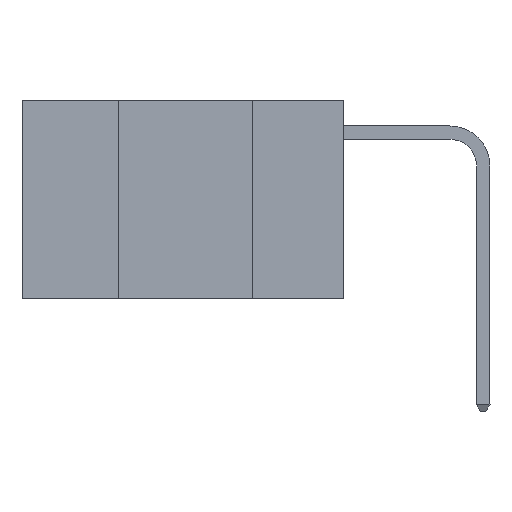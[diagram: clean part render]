
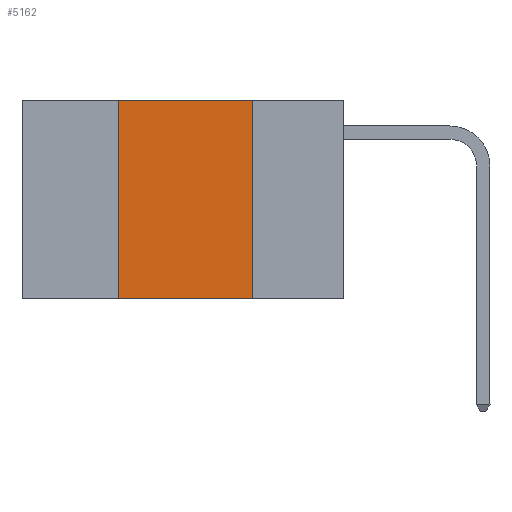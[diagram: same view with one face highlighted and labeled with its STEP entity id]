
A CAD part, left-side view. The second image highlights one B-rep face of the part: STEP entity #5162.
In plain terms, the highlighted planar face has unit normal (-1, 0, 0).
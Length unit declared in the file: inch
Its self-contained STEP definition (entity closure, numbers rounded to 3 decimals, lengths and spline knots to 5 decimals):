
#188 = EDGE_LOOP ( 'NONE', ( #9481, #11231, #2184, #12430 ) ) ;
#251 = CARTESIAN_POINT ( 'NONE',  ( 0., 0.6, -0.37 ) ) ;
#469 = DIRECTION ( 'NONE',  ( 0., 0., 1. ) ) ;
#737 = LINE ( 'NONE', #3701, #4433 ) ;
#960 = VERTEX_POINT ( 'NONE', #8768 ) ;
#1299 = CARTESIAN_POINT ( 'NONE',  ( 0., 0.42, 0. ) ) ;
#1723 = DIRECTION ( 'NONE',  ( 0., 0., -1. ) ) ;
#1767 = VECTOR ( 'NONE', #469, 39.37008 ) ;
#2184 = ORIENTED_EDGE ( 'NONE', *, *, #3793, .F. ) ;
#2724 = DIRECTION ( 'NONE',  ( 0., -1., 0. ) ) ;
#3566 = LINE ( 'NONE', #251, #10297 ) ;
#3701 = CARTESIAN_POINT ( 'NONE',  ( 0., 0.6, 0. ) ) ;
#3793 = EDGE_CURVE ( 'NONE', #13239, #7652, #7542, .T. ) ;
#3947 = CARTESIAN_POINT ( 'NONE',  ( 0., 0.42, -0.37 ) ) ;
#4055 = EDGE_CURVE ( 'NONE', #7652, #960, #737, .T. ) ;
#4138 = CARTESIAN_POINT ( 'NONE',  ( 0., 0.6, 0. ) ) ;
#4433 = VECTOR ( 'NONE', #2724, 39.37008 ) ;
#4456 = DIRECTION ( 'NONE',  ( 0., -1., 0. ) ) ;
#4818 = LINE ( 'NONE', #11314, #11617 ) ;
#5162 = ADVANCED_FACE ( 'NONE', ( #12511 ), #7145, .F. ) ;
#6239 = AXIS2_PLACEMENT_3D ( 'NONE', #4138, #13491, #9234 ) ;
#6911 = VERTEX_POINT ( 'NONE', #7906 ) ;
#7145 = PLANE ( 'NONE',  #6239 ) ;
#7542 = LINE ( 'NONE', #1299, #1767 ) ;
#7652 = VERTEX_POINT ( 'NONE', #8438 ) ;
#7906 = CARTESIAN_POINT ( 'NONE',  ( 0., 0.17, -0.37 ) ) ;
#8438 = CARTESIAN_POINT ( 'NONE',  ( 0., 0.42, 0. ) ) ;
#8768 = CARTESIAN_POINT ( 'NONE',  ( 0., 0.17, 0. ) ) ;
#9234 = DIRECTION ( 'NONE',  ( 0., 0., -1. ) ) ;
#9481 = ORIENTED_EDGE ( 'NONE', *, *, #13585, .F. ) ;
#10297 = VECTOR ( 'NONE', #4456, 39.37008 ) ;
#11231 = ORIENTED_EDGE ( 'NONE', *, *, #4055, .F. ) ;
#11314 = CARTESIAN_POINT ( 'NONE',  ( 0., 0.17, 0. ) ) ;
#11617 = VECTOR ( 'NONE', #1723, 39.37008 ) ;
#12430 = ORIENTED_EDGE ( 'NONE', *, *, #12562, .T. ) ;
#12511 = FACE_OUTER_BOUND ( 'NONE', #188, .T. ) ;
#12562 = EDGE_CURVE ( 'NONE', #13239, #6911, #3566, .T. ) ;
#13239 = VERTEX_POINT ( 'NONE', #3947 ) ;
#13491 = DIRECTION ( 'NONE',  ( 1., 0., 0. ) ) ;
#13585 = EDGE_CURVE ( 'NONE', #960, #6911, #4818, .T. ) ;
